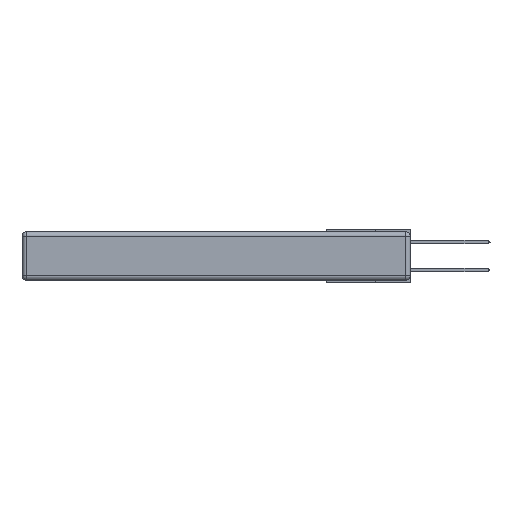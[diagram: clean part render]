
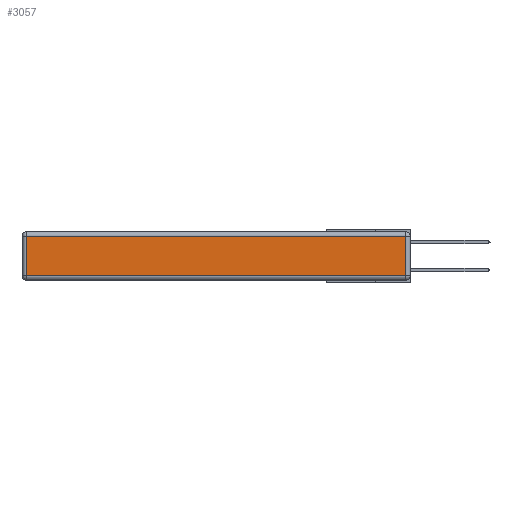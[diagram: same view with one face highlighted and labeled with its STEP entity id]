
A CAD part, left-side view. The second image highlights one B-rep face of the part: STEP entity #3057.
In plain terms, the highlighted planar face has unit normal (-1, 0, 0).
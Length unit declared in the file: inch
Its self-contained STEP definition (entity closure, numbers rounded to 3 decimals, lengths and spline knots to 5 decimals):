
#758 = VECTOR ( 'NONE', #20419, 39.37008 ) ;
#929 = LINE ( 'NONE', #5678, #18522 ) ;
#987 = ORIENTED_EDGE ( 'NONE', *, *, #6753, .T. ) ;
#1010 = LINE ( 'NONE', #9752, #11168 ) ;
#2741 = EDGE_LOOP ( 'NONE', ( #7460, #5643, #987, #6719 ) ) ;
#2946 = VERTEX_POINT ( 'NONE', #4346 ) ;
#3057 = ADVANCED_FACE ( 'NONE', ( #7070 ), #17132, .T. ) ;
#4220 = CARTESIAN_POINT ( 'NONE',  ( 0., 2.75, -0.03 ) ) ;
#4290 = DIRECTION ( 'NONE',  ( 0., 0., -1. ) ) ;
#4346 = CARTESIAN_POINT ( 'NONE',  ( 0., 0.03, -0.03 ) ) ;
#4612 = VERTEX_POINT ( 'NONE', #18312 ) ;
#4976 = AXIS2_PLACEMENT_3D ( 'NONE', #7659, #6280, #20330 ) ;
#5643 = ORIENTED_EDGE ( 'NONE', *, *, #11917, .T. ) ;
#5678 = CARTESIAN_POINT ( 'NONE',  ( 0., 2.72, -0.343 ) ) ;
#6280 = DIRECTION ( 'NONE',  ( -1., 0., 0. ) ) ;
#6372 = CARTESIAN_POINT ( 'NONE',  ( 0., 2.72, -0.313 ) ) ;
#6719 = ORIENTED_EDGE ( 'NONE', *, *, #11942, .T. ) ;
#6753 = EDGE_CURVE ( 'NONE', #2946, #4612, #7970, .T. ) ;
#7070 = FACE_OUTER_BOUND ( 'NONE', #2741, .T. ) ;
#7460 = ORIENTED_EDGE ( 'NONE', *, *, #11832, .T. ) ;
#7659 = CARTESIAN_POINT ( 'NONE',  ( 0., 0., -0.343 ) ) ;
#7970 = LINE ( 'NONE', #4220, #758 ) ;
#9752 = CARTESIAN_POINT ( 'NONE',  ( 0., 0., -0.313 ) ) ;
#11168 = VECTOR ( 'NONE', #13378, 39.37008 ) ;
#11363 = DIRECTION ( 'NONE',  ( 0., 0., 1. ) ) ;
#11832 = EDGE_CURVE ( 'NONE', #13606, #15952, #1010, .T. ) ;
#11917 = EDGE_CURVE ( 'NONE', #15952, #2946, #20438, .T. ) ;
#11942 = EDGE_CURVE ( 'NONE', #4612, #13606, #929, .T. ) ;
#13378 = DIRECTION ( 'NONE',  ( 0., -1., 0. ) ) ;
#13477 = CARTESIAN_POINT ( 'NONE',  ( 0., 0.03, -0.313 ) ) ;
#13606 = VERTEX_POINT ( 'NONE', #6372 ) ;
#14906 = CARTESIAN_POINT ( 'NONE',  ( 0., 0.03, -0.343 ) ) ;
#15952 = VERTEX_POINT ( 'NONE', #13477 ) ;
#17132 = PLANE ( 'NONE',  #4976 ) ;
#18312 = CARTESIAN_POINT ( 'NONE',  ( 0., 2.72, -0.03 ) ) ;
#18522 = VECTOR ( 'NONE', #4290, 39.37008 ) ;
#18676 = VECTOR ( 'NONE', #11363, 39.37008 ) ;
#20330 = DIRECTION ( 'NONE',  ( 0., 0., 1. ) ) ;
#20419 = DIRECTION ( 'NONE',  ( 0., 1., 0. ) ) ;
#20438 = LINE ( 'NONE', #14906, #18676 ) ;
